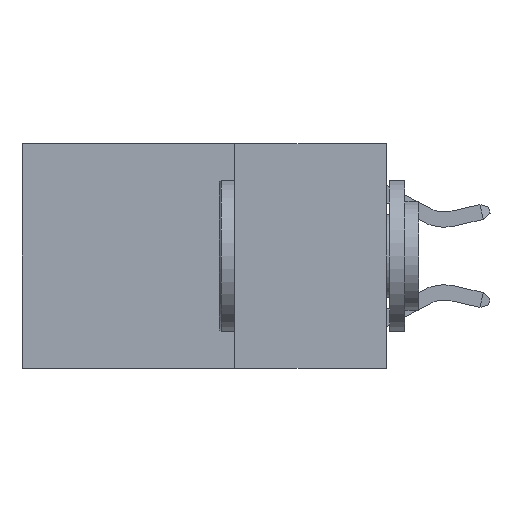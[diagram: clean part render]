
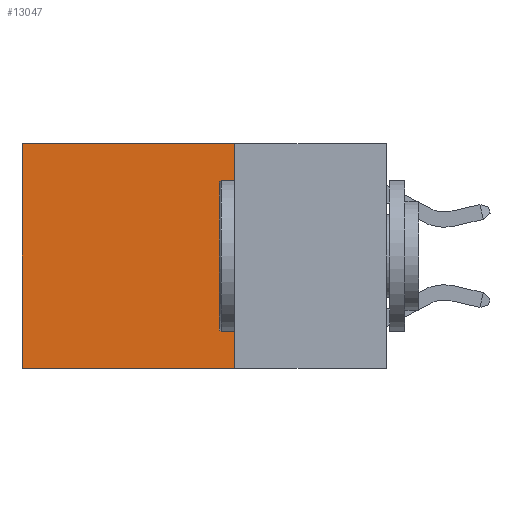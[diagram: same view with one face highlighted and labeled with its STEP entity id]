
A CAD part, left-side view. The second image highlights one B-rep face of the part: STEP entity #13047.
In plain terms, the highlighted planar face has unit normal (-1, 0, 0).
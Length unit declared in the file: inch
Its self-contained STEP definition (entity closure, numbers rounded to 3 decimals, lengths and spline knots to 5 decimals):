
#804 = ORIENTED_EDGE ( 'NONE', *, *, #10220, .T. ) ;
#1718 = VERTEX_POINT ( 'NONE', #8820 ) ;
#2932 = DIRECTION ( 'NONE',  ( 0., 0., -1. ) ) ;
#3138 = CARTESIAN_POINT ( 'NONE',  ( 0.2625, 0.25, 0. ) ) ;
#5511 = LINE ( 'NONE', #7620, #16626 ) ;
#6273 = CARTESIAN_POINT ( 'NONE',  ( 0.2625, 0.25, 0. ) ) ;
#7620 = CARTESIAN_POINT ( 'NONE',  ( 0.2625, 0.25, 0. ) ) ;
#7779 = ORIENTED_EDGE ( 'NONE', *, *, #26374, .F. ) ;
#8184 = LINE ( 'NONE', #20510, #19267 ) ;
#8486 = DIRECTION ( 'NONE',  ( 0., 0., -1. ) ) ;
#8820 = CARTESIAN_POINT ( 'NONE',  ( 0.2625, 0.25, -0.37 ) ) ;
#8861 = ORIENTED_EDGE ( 'NONE', *, *, #19411, .T. ) ;
#8904 = ORIENTED_EDGE ( 'NONE', *, *, #27888, .F. ) ;
#8990 = CARTESIAN_POINT ( 'NONE',  ( 0.2625, 0.6, 0. ) ) ;
#10220 = EDGE_CURVE ( 'NONE', #10933, #21231, #5511, .T. ) ;
#10545 = VECTOR ( 'NONE', #13202, 39.37008 ) ;
#10560 = FACE_OUTER_BOUND ( 'NONE', #24561, .T. ) ;
#10933 = VERTEX_POINT ( 'NONE', #3138 ) ;
#11879 = VECTOR ( 'NONE', #2932, 39.37008 ) ;
#13047 = ADVANCED_FACE ( 'NONE', ( #10560 ), #15083, .F. ) ;
#13202 = DIRECTION ( 'NONE',  ( 0., 1., 0. ) ) ;
#13826 = VERTEX_POINT ( 'NONE', #15234 ) ;
#14326 = DIRECTION ( 'NONE',  ( 0., 1., 0. ) ) ;
#15083 = PLANE ( 'NONE',  #18325 ) ;
#15234 = CARTESIAN_POINT ( 'NONE',  ( 0.2625, 0.6, -0.37 ) ) ;
#16626 = VECTOR ( 'NONE', #14326, 39.37008 ) ;
#18325 = AXIS2_PLACEMENT_3D ( 'NONE', #6273, #21612, #8486 ) ;
#18455 = CARTESIAN_POINT ( 'NONE',  ( 0.2625, 0.25, 0. ) ) ;
#19267 = VECTOR ( 'NONE', #22616, 39.37008 ) ;
#19411 = EDGE_CURVE ( 'NONE', #21231, #13826, #8184, .T. ) ;
#19732 = CARTESIAN_POINT ( 'NONE',  ( 0.2625, 0.25, -0.37 ) ) ;
#20510 = CARTESIAN_POINT ( 'NONE',  ( 0.2625, 0.6, 0. ) ) ;
#21231 = VERTEX_POINT ( 'NONE', #8990 ) ;
#21612 = DIRECTION ( 'NONE',  ( 1., 0., 0. ) ) ;
#22616 = DIRECTION ( 'NONE',  ( 0., 0., -1. ) ) ;
#22747 = LINE ( 'NONE', #18455, #11879 ) ;
#22796 = LINE ( 'NONE', #19732, #10545 ) ;
#24561 = EDGE_LOOP ( 'NONE', ( #8861, #7779, #8904, #804 ) ) ;
#26374 = EDGE_CURVE ( 'NONE', #1718, #13826, #22796, .T. ) ;
#27888 = EDGE_CURVE ( 'NONE', #10933, #1718, #22747, .T. ) ;
